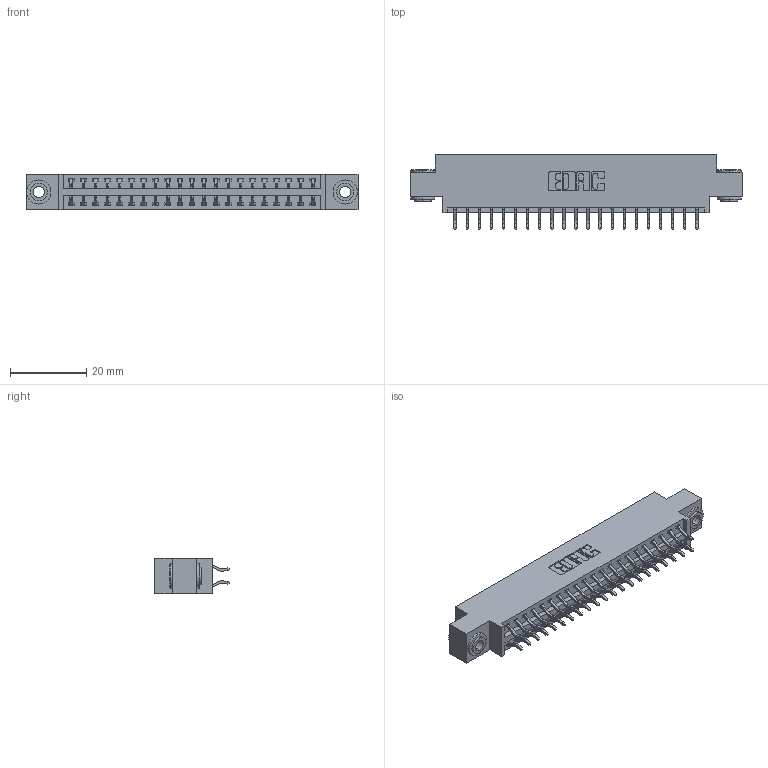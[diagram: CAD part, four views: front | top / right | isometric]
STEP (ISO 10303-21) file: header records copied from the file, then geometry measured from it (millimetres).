
FILE_DESCRIPTION (( 'STEP AP203' ), '1' );
FILE_NAME ('396-042-556-803.STEP', '2018-09-07T01:03:29', ( '' ), ( '' ), 'SwSTEP 2.0', 'SolidWorks 2016', '' );
FILE_SCHEMA (( 'CONFIG_CONTROL_DESIGN' ));
Length unit declared in the file: inch
Products named in the file (4): 345-250-002_345-250-002-102; 396-042-556-803; 346 Part_0.170 Offset - 0.156 Dia-TH; 345-292-001_556 Tail
Assembly tree (45 placements, depth 2):
  396-042-556-803
    346 Part_0.170 Offset - 0.156 Dia-TH
    345-292-001_556 Tail  x42
    345-250-002_345-250-002-102  x2
Bounding box: 87.25 x 19.57 x 9.4 mm (x, y, z)
Volume: 8207.9 mm3; surface area: 11307 mm2
Topology: 45 solids, 45 shells, 2600 faces, 7683 edges, 5062 vertices
Faces by surface type: plane 1728, cylinder 864, cone 8
Entity records: 17534 total; most frequent: CARTESIAN_POINT 2911, ORIENTED_EDGE 2826, DIRECTION 2635, EDGE_CURVE 1413, LINE 1165, VECTOR 1165, VERTEX_POINT 938, AXIS2_PLACEMENT_3D 735
